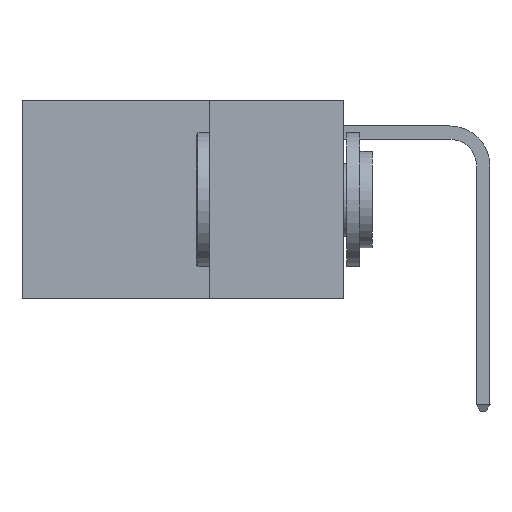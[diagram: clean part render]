
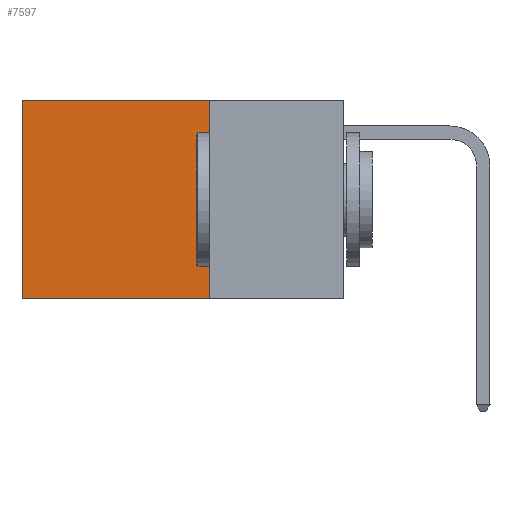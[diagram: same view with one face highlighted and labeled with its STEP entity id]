
A CAD part, left-side view. The second image highlights one B-rep face of the part: STEP entity #7597.
In plain terms, the highlighted planar face has unit normal (-1, 0, 0).
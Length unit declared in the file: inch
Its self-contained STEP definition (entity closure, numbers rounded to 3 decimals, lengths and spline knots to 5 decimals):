
#141 = DIRECTION ( 'NONE',  ( 0., 0., -1. ) ) ;
#302 = DIRECTION ( 'NONE',  ( 0., 0., -1. ) ) ;
#340 = EDGE_CURVE ( 'NONE', #5961, #6726, #756, .T. ) ;
#439 = CARTESIAN_POINT ( 'NONE',  ( 0.2625, 0.25, 0. ) ) ;
#491 = CARTESIAN_POINT ( 'NONE',  ( 0.2625, 0.25, 0. ) ) ;
#756 = LINE ( 'NONE', #3996, #9769 ) ;
#1123 = CARTESIAN_POINT ( 'NONE',  ( 0.2625, 0.25, 0. ) ) ;
#1195 = EDGE_LOOP ( 'NONE', ( #10231, #5363, #10860, #4970 ) ) ;
#1433 = EDGE_CURVE ( 'NONE', #6726, #6610, #8124, .T. ) ;
#1530 = VECTOR ( 'NONE', #4818, 39.37008 ) ;
#1776 = VERTEX_POINT ( 'NONE', #10328 ) ;
#2005 = DIRECTION ( 'NONE',  ( 1., 0., 0. ) ) ;
#2680 = LINE ( 'NONE', #5533, #7048 ) ;
#3605 = CARTESIAN_POINT ( 'NONE',  ( 0.2625, 0.25, -0.37 ) ) ;
#3996 = CARTESIAN_POINT ( 'NONE',  ( 0.2625, 0.25, 0. ) ) ;
#4818 = DIRECTION ( 'NONE',  ( 0., 1., 0. ) ) ;
#4970 = ORIENTED_EDGE ( 'NONE', *, *, #10138, .T. ) ;
#5359 = DIRECTION ( 'NONE',  ( 0., 1., 0. ) ) ;
#5363 = ORIENTED_EDGE ( 'NONE', *, *, #1433, .F. ) ;
#5533 = CARTESIAN_POINT ( 'NONE',  ( 0.2625, 0.6, 0. ) ) ;
#5722 = CARTESIAN_POINT ( 'NONE',  ( 0.2625, 0.6, -0.37 ) ) ;
#5961 = VERTEX_POINT ( 'NONE', #491 ) ;
#6352 = PLANE ( 'NONE',  #8729 ) ;
#6610 = VERTEX_POINT ( 'NONE', #5722 ) ;
#6720 = LINE ( 'NONE', #439, #1530 ) ;
#6726 = VERTEX_POINT ( 'NONE', #10188 ) ;
#7048 = VECTOR ( 'NONE', #302, 39.37008 ) ;
#7597 = ADVANCED_FACE ( 'NONE', ( #8415 ), #6352, .F. ) ;
#8104 = DIRECTION ( 'NONE',  ( 0., 0., -1. ) ) ;
#8124 = LINE ( 'NONE', #3605, #10423 ) ;
#8217 = EDGE_CURVE ( 'NONE', #1776, #6610, #2680, .T. ) ;
#8415 = FACE_OUTER_BOUND ( 'NONE', #1195, .T. ) ;
#8729 = AXIS2_PLACEMENT_3D ( 'NONE', #1123, #2005, #8104 ) ;
#9769 = VECTOR ( 'NONE', #141, 39.37008 ) ;
#10138 = EDGE_CURVE ( 'NONE', #5961, #1776, #6720, .T. ) ;
#10188 = CARTESIAN_POINT ( 'NONE',  ( 0.2625, 0.25, -0.37 ) ) ;
#10231 = ORIENTED_EDGE ( 'NONE', *, *, #8217, .T. ) ;
#10328 = CARTESIAN_POINT ( 'NONE',  ( 0.2625, 0.6, 0. ) ) ;
#10423 = VECTOR ( 'NONE', #5359, 39.37008 ) ;
#10860 = ORIENTED_EDGE ( 'NONE', *, *, #340, .F. ) ;
